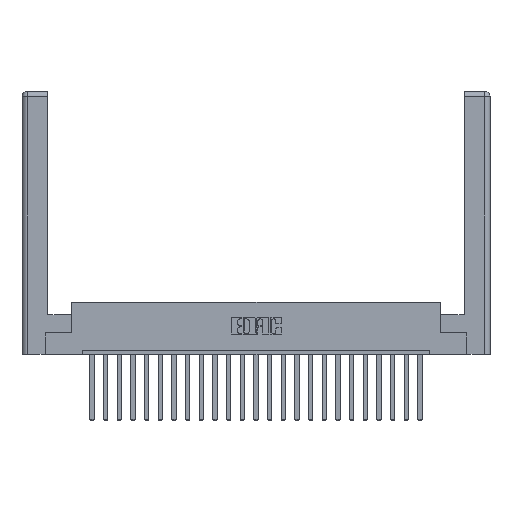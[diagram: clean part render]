
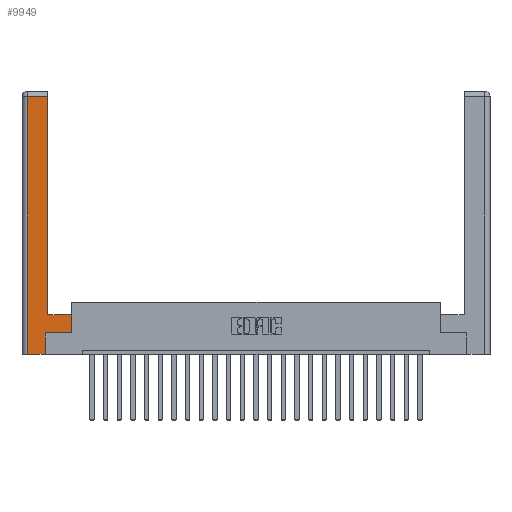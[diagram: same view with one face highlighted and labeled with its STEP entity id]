
A CAD part, top view. The second image highlights one B-rep face of the part: STEP entity #9949.
In plain terms, the highlighted planar face has unit normal (0, 0, 1).
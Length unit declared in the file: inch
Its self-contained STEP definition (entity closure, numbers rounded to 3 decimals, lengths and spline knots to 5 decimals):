
#25 = LINE ( 'NONE', #6574, #5380 ) ;
#492 = VECTOR ( 'NONE', #14987, 39.37008 ) ;
#1219 = ORIENTED_EDGE ( 'NONE', *, *, #10223, .T. ) ;
#2197 = DIRECTION ( 'NONE',  ( 0., -1., 0. ) ) ;
#2245 = LINE ( 'NONE', #7706, #9214 ) ;
#2283 = CARTESIAN_POINT ( 'NONE',  ( 0.295, 0.45, 0. ) ) ;
#3301 = DIRECTION ( 'NONE',  ( 0., 1., 0. ) ) ;
#3493 = VERTEX_POINT ( 'NONE', #22561 ) ;
#4414 = LINE ( 'NONE', #18781, #20106 ) ;
#4811 = ORIENTED_EDGE ( 'NONE', *, *, #13527, .T. ) ;
#4911 = ORIENTED_EDGE ( 'NONE', *, *, #13801, .T. ) ;
#5118 = CARTESIAN_POINT ( 'NONE',  ( 0.265, 0., 0. ) ) ;
#5380 = VECTOR ( 'NONE', #10384, 39.37008 ) ;
#5788 = ORIENTED_EDGE ( 'NONE', *, *, #15717, .T. ) ;
#6190 = DIRECTION ( 'NONE',  ( 0., 1., 0. ) ) ;
#6203 = CARTESIAN_POINT ( 'NONE',  ( 0.0615, 2.94, 0. ) ) ;
#6487 = LINE ( 'NONE', #21597, #8414 ) ;
#6574 = CARTESIAN_POINT ( 'NONE',  ( 0.295, 0.45, 0. ) ) ;
#6722 = EDGE_CURVE ( 'NONE', #17005, #3493, #17881, .T. ) ;
#6725 = ORIENTED_EDGE ( 'NONE', *, *, #15747, .T. ) ;
#7641 = ORIENTED_EDGE ( 'NONE', *, *, #13451, .T. ) ;
#7706 = CARTESIAN_POINT ( 'NONE',  ( 0.565, 0.245, 0. ) ) ;
#8324 = EDGE_LOOP ( 'NONE', ( #6725, #9085, #5788, #4811, #7641, #4911, #1219, #10152 ) ) ;
#8414 = VECTOR ( 'NONE', #18544, 39.37008 ) ;
#9085 = ORIENTED_EDGE ( 'NONE', *, *, #6722, .T. ) ;
#9214 = VECTOR ( 'NONE', #13328, 39.37008 ) ;
#9285 = CARTESIAN_POINT ( 'NONE',  ( 0.0615, 0., 0. ) ) ;
#9362 = CARTESIAN_POINT ( 'NONE',  ( 0.0615, 0., 0. ) ) ;
#9789 = LINE ( 'NONE', #10429, #18508 ) ;
#9949 = ADVANCED_FACE ( 'NONE', ( #12331 ), #18919, .F. ) ;
#10007 = CARTESIAN_POINT ( 'NONE',  ( 0.295, 2.94, 0. ) ) ;
#10152 = ORIENTED_EDGE ( 'NONE', *, *, #13026, .T. ) ;
#10223 = EDGE_CURVE ( 'NONE', #17174, #17516, #6487, .T. ) ;
#10384 = DIRECTION ( 'NONE',  ( -1., 0., 0. ) ) ;
#10429 = CARTESIAN_POINT ( 'NONE',  ( 0.265, 0.245, 0. ) ) ;
#10840 = VECTOR ( 'NONE', #2197, 39.37008 ) ;
#12331 = FACE_OUTER_BOUND ( 'NONE', #8324, .T. ) ;
#13026 = EDGE_CURVE ( 'NONE', #17516, #21041, #25, .T. ) ;
#13328 = DIRECTION ( 'NONE',  ( 1., 0., 0. ) ) ;
#13361 = DIRECTION ( 'NONE',  ( 0., 0., -1. ) ) ;
#13451 = EDGE_CURVE ( 'NONE', #21164, #14729, #9789, .T. ) ;
#13527 = EDGE_CURVE ( 'NONE', #18714, #21164, #13734, .T. ) ;
#13670 = DIRECTION ( 'NONE',  ( -1., 0., 0. ) ) ;
#13734 = LINE ( 'NONE', #5118, #16577 ) ;
#13801 = EDGE_CURVE ( 'NONE', #14729, #17174, #2245, .T. ) ;
#13806 = DIRECTION ( 'NONE',  ( 1., 0., 0. ) ) ;
#14021 = CARTESIAN_POINT ( 'NONE',  ( 0.565, 0.245, 0. ) ) ;
#14092 = AXIS2_PLACEMENT_3D ( 'NONE', #20730, #13361, #13670 ) ;
#14729 = VERTEX_POINT ( 'NONE', #19016 ) ;
#14987 = DIRECTION ( 'NONE',  ( -1., 0., 0. ) ) ;
#15717 = EDGE_CURVE ( 'NONE', #3493, #18714, #17077, .T. ) ;
#15747 = EDGE_CURVE ( 'NONE', #21041, #17005, #4414, .T. ) ;
#16577 = VECTOR ( 'NONE', #13806, 39.37008 ) ;
#17005 = VERTEX_POINT ( 'NONE', #10007 ) ;
#17077 = LINE ( 'NONE', #9285, #10840 ) ;
#17103 = CARTESIAN_POINT ( 'NONE',  ( 0.265, 0., 0. ) ) ;
#17174 = VERTEX_POINT ( 'NONE', #14021 ) ;
#17516 = VERTEX_POINT ( 'NONE', #17577 ) ;
#17577 = CARTESIAN_POINT ( 'NONE',  ( 0.565, 0.45, 0. ) ) ;
#17881 = LINE ( 'NONE', #6203, #492 ) ;
#18508 = VECTOR ( 'NONE', #3301, 39.37008 ) ;
#18544 = DIRECTION ( 'NONE',  ( 0., 1., 0. ) ) ;
#18714 = VERTEX_POINT ( 'NONE', #9362 ) ;
#18781 = CARTESIAN_POINT ( 'NONE',  ( 0.295, 3., 0. ) ) ;
#18919 = PLANE ( 'NONE',  #14092 ) ;
#19016 = CARTESIAN_POINT ( 'NONE',  ( 0.265, 0.245, 0. ) ) ;
#20106 = VECTOR ( 'NONE', #6190, 39.37008 ) ;
#20730 = CARTESIAN_POINT ( 'NONE',  ( 0., 0., 0. ) ) ;
#21041 = VERTEX_POINT ( 'NONE', #2283 ) ;
#21164 = VERTEX_POINT ( 'NONE', #17103 ) ;
#21597 = CARTESIAN_POINT ( 'NONE',  ( 0.565, 0.45, 0. ) ) ;
#22561 = CARTESIAN_POINT ( 'NONE',  ( 0.0615, 2.94, 0. ) ) ;
